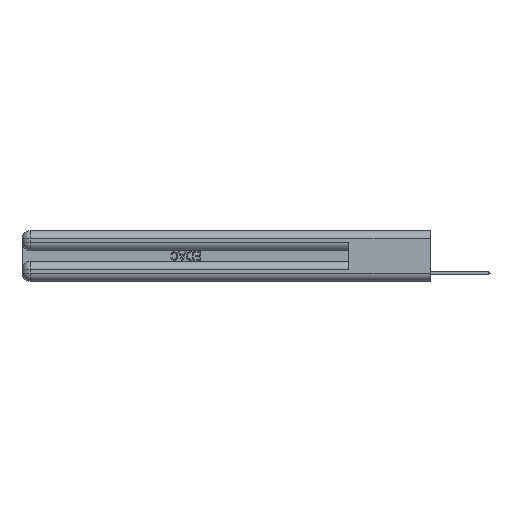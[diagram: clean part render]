
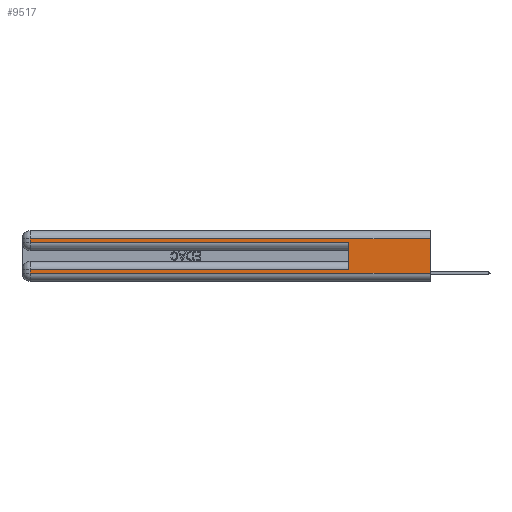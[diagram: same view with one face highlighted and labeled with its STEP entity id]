
A CAD part, left-side view. The second image highlights one B-rep face of the part: STEP entity #9517.
In plain terms, the highlighted planar face has unit normal (-1, 0, 0).
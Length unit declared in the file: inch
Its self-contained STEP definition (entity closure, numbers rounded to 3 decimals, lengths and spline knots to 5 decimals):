
#176 = PLANE ( 'NONE',  #24038 ) ;
#706 = CARTESIAN_POINT ( 'NONE',  ( 0., 0., 0.06 ) ) ;
#865 = VERTEX_POINT ( 'NONE', #706 ) ;
#1144 = CARTESIAN_POINT ( 'NONE',  ( 0., 2.94, 0.06 ) ) ;
#1579 = EDGE_CURVE ( 'NONE', #5815, #10937, #19607, .T. ) ;
#2083 = DIRECTION ( 'NONE',  ( 1., 0., 0. ) ) ;
#2408 = VERTEX_POINT ( 'NONE', #9729 ) ;
#2923 = CARTESIAN_POINT ( 'NONE',  ( 0., 0., 0.085 ) ) ;
#2955 = DIRECTION ( 'NONE',  ( 0., -1., 0. ) ) ;
#3029 = ORIENTED_EDGE ( 'NONE', *, *, #1579, .T. ) ;
#3898 = ORIENTED_EDGE ( 'NONE', *, *, #4705, .F. ) ;
#4419 = ORIENTED_EDGE ( 'NONE', *, *, #8231, .T. ) ;
#4690 = CARTESIAN_POINT ( 'NONE',  ( 0., 0.6, 0.145 ) ) ;
#4705 = EDGE_CURVE ( 'NONE', #33372, #2408, #32828, .T. ) ;
#4719 = CARTESIAN_POINT ( 'NONE',  ( 0., 2.94, 0.085 ) ) ;
#4893 = ORIENTED_EDGE ( 'NONE', *, *, #31881, .T. ) ;
#5545 = ORIENTED_EDGE ( 'NONE', *, *, #13194, .T. ) ;
#5815 = VERTEX_POINT ( 'NONE', #27045 ) ;
#6306 = LINE ( 'NONE', #26302, #30943 ) ;
#8231 = EDGE_CURVE ( 'NONE', #33372, #32831, #26275, .T. ) ;
#8264 = CARTESIAN_POINT ( 'NONE',  ( 0., 0., 0.285 ) ) ;
#9292 = DIRECTION ( 'NONE',  ( 0., 0., 1. ) ) ;
#9517 = ADVANCED_FACE ( 'NONE', ( #13099 ), #176, .F. ) ;
#9729 = CARTESIAN_POINT ( 'NONE',  ( 0., 0.6, 0.285 ) ) ;
#10009 = CARTESIAN_POINT ( 'NONE',  ( 0., 0.6, 0.085 ) ) ;
#10408 = CARTESIAN_POINT ( 'NONE',  ( 0., 2.94, 0.31 ) ) ;
#10598 = LINE ( 'NONE', #23902, #19466 ) ;
#10839 = ORIENTED_EDGE ( 'NONE', *, *, #28347, .T. ) ;
#10890 = VECTOR ( 'NONE', #23699, 39.37008 ) ;
#10937 = VERTEX_POINT ( 'NONE', #10408 ) ;
#11557 = CARTESIAN_POINT ( 'NONE',  ( 0., 2.94, 0.285 ) ) ;
#11613 = LINE ( 'NONE', #11944, #16636 ) ;
#11944 = CARTESIAN_POINT ( 'NONE',  ( 0., 0., 0.37 ) ) ;
#12216 = EDGE_LOOP ( 'NONE', ( #28409, #3029, #10839, #5545, #3898, #4419, #4893, #21213 ) ) ;
#12459 = CARTESIAN_POINT ( 'NONE',  ( 0., 2.94, 0.37 ) ) ;
#12531 = VERTEX_POINT ( 'NONE', #11557 ) ;
#13099 = FACE_OUTER_BOUND ( 'NONE', #12216, .T. ) ;
#13194 = EDGE_CURVE ( 'NONE', #12531, #2408, #23785, .T. ) ;
#13456 = VERTEX_POINT ( 'NONE', #1144 ) ;
#14981 = DIRECTION ( 'NONE',  ( 0., 1., 0. ) ) ;
#15549 = DIRECTION ( 'NONE',  ( 0., 0., -1. ) ) ;
#16481 = DIRECTION ( 'NONE',  ( 0., -1., 0. ) ) ;
#16636 = VECTOR ( 'NONE', #20125, 39.37008 ) ;
#19466 = VECTOR ( 'NONE', #15549, 39.37008 ) ;
#19473 = VECTOR ( 'NONE', #9292, 39.37008 ) ;
#19607 = LINE ( 'NONE', #27606, #23483 ) ;
#20125 = DIRECTION ( 'NONE',  ( 0., 0., -1. ) ) ;
#20398 = VECTOR ( 'NONE', #16481, 39.37008 ) ;
#21213 = ORIENTED_EDGE ( 'NONE', *, *, #29033, .T. ) ;
#23483 = VECTOR ( 'NONE', #14981, 39.37008 ) ;
#23699 = DIRECTION ( 'NONE',  ( 0., 1., 0. ) ) ;
#23785 = LINE ( 'NONE', #8264, #20398 ) ;
#23902 = CARTESIAN_POINT ( 'NONE',  ( 0., 2.94, 0.37 ) ) ;
#24038 = AXIS2_PLACEMENT_3D ( 'NONE', #26229, #2083, #25262 ) ;
#24988 = VECTOR ( 'NONE', #28156, 39.37008 ) ;
#25262 = DIRECTION ( 'NONE',  ( 0., 0., -1. ) ) ;
#25740 = EDGE_CURVE ( 'NONE', #5815, #865, #11613, .T. ) ;
#26229 = CARTESIAN_POINT ( 'NONE',  ( 0., 0., 0.37 ) ) ;
#26275 = LINE ( 'NONE', #2923, #10890 ) ;
#26302 = CARTESIAN_POINT ( 'NONE',  ( 0., 0., 0.06 ) ) ;
#27045 = CARTESIAN_POINT ( 'NONE',  ( 0., 0., 0.31 ) ) ;
#27606 = CARTESIAN_POINT ( 'NONE',  ( 0., 0., 0.31 ) ) ;
#28156 = DIRECTION ( 'NONE',  ( 0., 0., -1. ) ) ;
#28347 = EDGE_CURVE ( 'NONE', #10937, #12531, #10598, .T. ) ;
#28409 = ORIENTED_EDGE ( 'NONE', *, *, #25740, .F. ) ;
#29033 = EDGE_CURVE ( 'NONE', #13456, #865, #6306, .T. ) ;
#30869 = LINE ( 'NONE', #12459, #24988 ) ;
#30943 = VECTOR ( 'NONE', #2955, 39.37008 ) ;
#31881 = EDGE_CURVE ( 'NONE', #32831, #13456, #30869, .T. ) ;
#32828 = LINE ( 'NONE', #4690, #19473 ) ;
#32831 = VERTEX_POINT ( 'NONE', #4719 ) ;
#33372 = VERTEX_POINT ( 'NONE', #10009 ) ;
